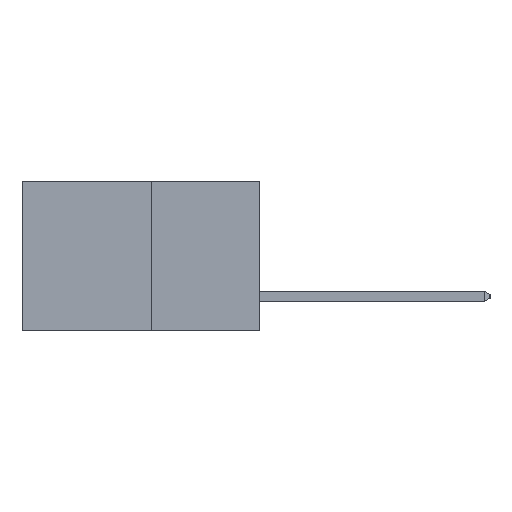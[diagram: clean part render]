
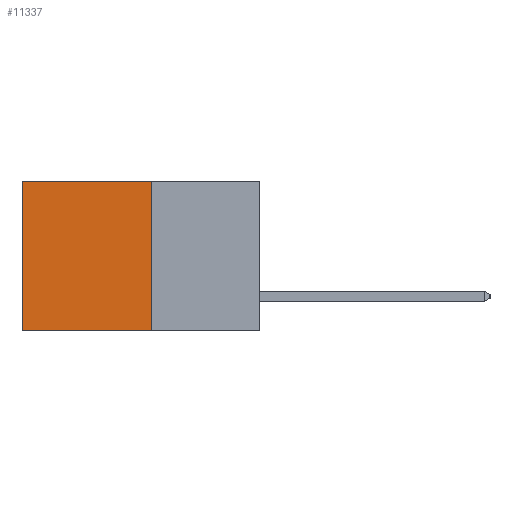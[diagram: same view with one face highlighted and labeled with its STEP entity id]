
A CAD part, left-side view. The second image highlights one B-rep face of the part: STEP entity #11337.
In plain terms, the highlighted planar face has unit normal (-1, 0, 0).
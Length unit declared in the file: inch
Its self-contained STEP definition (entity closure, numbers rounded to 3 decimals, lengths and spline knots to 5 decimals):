
#365 = EDGE_CURVE ( 'NONE', #2266, #10772, #2601, .T. ) ;
#430 = DIRECTION ( 'NONE',  ( 0., 1., 0. ) ) ;
#469 = EDGE_CURVE ( 'NONE', #2710, #2266, #4363, .T. ) ;
#768 = DIRECTION ( 'NONE',  ( 0., 0., -1. ) ) ;
#1263 = CARTESIAN_POINT ( 'NONE',  ( 0.277, 0.27, -0.37 ) ) ;
#1347 = EDGE_LOOP ( 'NONE', ( #1632, #2857, #5984, #9793 ) ) ;
#1632 = ORIENTED_EDGE ( 'NONE', *, *, #365, .T. ) ;
#1662 = CARTESIAN_POINT ( 'NONE',  ( 0.277, 0.27, 0. ) ) ;
#1866 = VECTOR ( 'NONE', #8792, 39.37008 ) ;
#2266 = VERTEX_POINT ( 'NONE', #6865 ) ;
#2601 = LINE ( 'NONE', #11187, #7885 ) ;
#2621 = CARTESIAN_POINT ( 'NONE',  ( 0.277, 0.27, 0. ) ) ;
#2710 = VERTEX_POINT ( 'NONE', #2621 ) ;
#2774 = EDGE_CURVE ( 'NONE', #8937, #10772, #8875, .T. ) ;
#2857 = ORIENTED_EDGE ( 'NONE', *, *, #2774, .F. ) ;
#3617 = FACE_OUTER_BOUND ( 'NONE', #1347, .T. ) ;
#4311 = EDGE_CURVE ( 'NONE', #2710, #8937, #12177, .T. ) ;
#4363 = LINE ( 'NONE', #1662, #9223 ) ;
#5362 = CARTESIAN_POINT ( 'NONE',  ( 0.277, 0.59, -0.37 ) ) ;
#5984 = ORIENTED_EDGE ( 'NONE', *, *, #4311, .F. ) ;
#6140 = CARTESIAN_POINT ( 'NONE',  ( 0.277, 0.27, -0.37 ) ) ;
#6643 = DIRECTION ( 'NONE',  ( 0., 1., 0. ) ) ;
#6865 = CARTESIAN_POINT ( 'NONE',  ( 0.277, 0.59, 0. ) ) ;
#7885 = VECTOR ( 'NONE', #12346, 39.37008 ) ;
#7973 = VECTOR ( 'NONE', #430, 39.37008 ) ;
#8792 = DIRECTION ( 'NONE',  ( 0., 0., -1. ) ) ;
#8875 = LINE ( 'NONE', #1263, #7973 ) ;
#8937 = VERTEX_POINT ( 'NONE', #10058 ) ;
#9223 = VECTOR ( 'NONE', #6643, 39.37008 ) ;
#9667 = DIRECTION ( 'NONE',  ( 1., 0., 0. ) ) ;
#9793 = ORIENTED_EDGE ( 'NONE', *, *, #469, .T. ) ;
#10058 = CARTESIAN_POINT ( 'NONE',  ( 0.277, 0.27, -0.37 ) ) ;
#10167 = AXIS2_PLACEMENT_3D ( 'NONE', #11525, #9667, #768 ) ;
#10772 = VERTEX_POINT ( 'NONE', #5362 ) ;
#11187 = CARTESIAN_POINT ( 'NONE',  ( 0.277, 0.59, -0.37 ) ) ;
#11337 = ADVANCED_FACE ( 'NONE', ( #3617 ), #12482, .F. ) ;
#11525 = CARTESIAN_POINT ( 'NONE',  ( 0.277, 0.27, -0.37 ) ) ;
#12177 = LINE ( 'NONE', #6140, #1866 ) ;
#12346 = DIRECTION ( 'NONE',  ( 0., 0., -1. ) ) ;
#12482 = PLANE ( 'NONE',  #10167 ) ;
